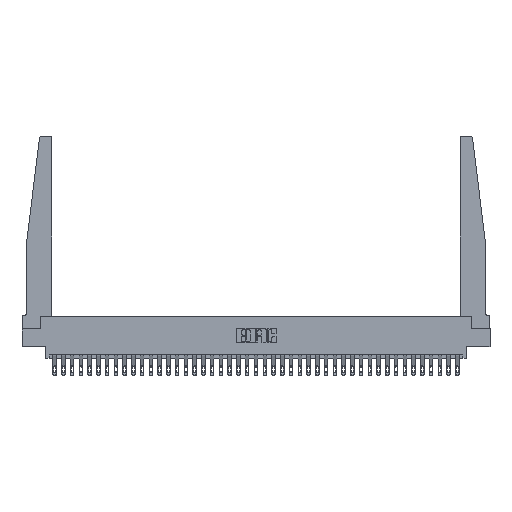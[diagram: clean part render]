
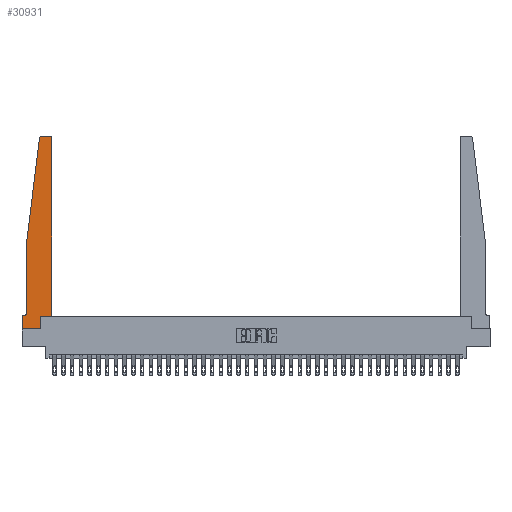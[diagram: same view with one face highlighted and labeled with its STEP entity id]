
A CAD part, top view. The second image highlights one B-rep face of the part: STEP entity #30931.
In plain terms, the highlighted planar face has unit normal (0, 0, 1).
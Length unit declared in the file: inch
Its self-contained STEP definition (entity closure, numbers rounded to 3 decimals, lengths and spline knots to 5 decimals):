
#15 = ORIENTED_EDGE ( 'NONE', *, *, #18158, .T. ) ;
#240 = CARTESIAN_POINT ( 'NONE',  ( 0.015, 0.1875, 0.37 ) ) ;
#289 = DIRECTION ( 'NONE',  ( 1., 0., 0. ) ) ;
#317 = CARTESIAN_POINT ( 'NONE',  ( 0.27653, 2.75, 0.37 ) ) ;
#432 = LINE ( 'NONE', #13810, #22222 ) ;
#491 = DIRECTION ( 'NONE',  ( 0., 0., 1. ) ) ;
#608 = EDGE_LOOP ( 'NONE', ( #12430, #9881, #7657, #9172, #32978, #2568, #4716, #7110, #5263, #15, #32462, #26759 ) ) ;
#674 = EDGE_CURVE ( 'NONE', #17049, #8147, #21334, .T. ) ;
#1508 = EDGE_CURVE ( 'NONE', #14653, #20918, #10720, .T. ) ;
#2113 = DIRECTION ( 'NONE',  ( -0.122, -0.992, 0. ) ) ;
#2166 = VECTOR ( 'NONE', #9971, 39.37008 ) ;
#2568 = ORIENTED_EDGE ( 'NONE', *, *, #34248, .T. ) ;
#2602 = EDGE_CURVE ( 'NONE', #24533, #17049, #34539, .T. ) ;
#2658 = DIRECTION ( 'NONE',  ( 0., 0., 1. ) ) ;
#4085 = VERTEX_POINT ( 'NONE', #24795 ) ;
#4716 = ORIENTED_EDGE ( 'NONE', *, *, #15577, .T. ) ;
#4764 = EDGE_CURVE ( 'NONE', #12206, #24533, #18364, .T. ) ;
#4895 = VECTOR ( 'NONE', #10423, 39.37008 ) ;
#5263 = ORIENTED_EDGE ( 'NONE', *, *, #34010, .T. ) ;
#5639 = CIRCLE ( 'NONE', #25827, 0.03 ) ;
#7110 = ORIENTED_EDGE ( 'NONE', *, *, #1508, .T. ) ;
#7355 = DIRECTION ( 'NONE',  ( 1., 0., 0. ) ) ;
#7657 = ORIENTED_EDGE ( 'NONE', *, *, #29486, .T. ) ;
#8147 = VERTEX_POINT ( 'NONE', #317 ) ;
#8255 = FACE_OUTER_BOUND ( 'NONE', #608, .T. ) ;
#8625 = CARTESIAN_POINT ( 'NONE',  ( 0., 0., 0.37 ) ) ;
#8707 = VECTOR ( 'NONE', #2113, 39.37008 ) ;
#9172 = ORIENTED_EDGE ( 'NONE', *, *, #20859, .T. ) ;
#9446 = CARTESIAN_POINT ( 'NONE',  ( 0.395, 2.75, 0.37 ) ) ;
#9881 = ORIENTED_EDGE ( 'NONE', *, *, #22931, .T. ) ;
#9971 = DIRECTION ( 'NONE',  ( -1., 0., 0. ) ) ;
#10423 = DIRECTION ( 'NONE',  ( 0., 1., 0. ) ) ;
#10720 = LINE ( 'NONE', #26637, #19489 ) ;
#12206 = VERTEX_POINT ( 'NONE', #17383 ) ;
#12224 = DIRECTION ( 'NONE',  ( 0., 0., 1. ) ) ;
#12430 = ORIENTED_EDGE ( 'NONE', *, *, #674, .T. ) ;
#13709 = VECTOR ( 'NONE', #29990, 39.37008 ) ;
#13810 = CARTESIAN_POINT ( 'NONE',  ( 0.425, 0.18, 0.37 ) ) ;
#13817 = VERTEX_POINT ( 'NONE', #22106 ) ;
#13925 = VECTOR ( 'NONE', #26921, 39.37008 ) ;
#14653 = VERTEX_POINT ( 'NONE', #8625 ) ;
#15577 = EDGE_CURVE ( 'NONE', #21917, #14653, #30214, .T. ) ;
#15705 = LINE ( 'NONE', #29074, #13925 ) ;
#16513 = LINE ( 'NONE', #25017, #29810 ) ;
#16714 = CARTESIAN_POINT ( 'NONE',  ( 0.24675, 2.72367, 0.37 ) ) ;
#16725 = CARTESIAN_POINT ( 'NONE',  ( 0., 0.1875, 0.37 ) ) ;
#17049 = VERTEX_POINT ( 'NONE', #9446 ) ;
#17383 = CARTESIAN_POINT ( 'NONE',  ( 0.425, 0.18, 0.37 ) ) ;
#18064 = VECTOR ( 'NONE', #19045, 39.37008 ) ;
#18158 = EDGE_CURVE ( 'NONE', #13817, #12206, #432, .T. ) ;
#18364 = LINE ( 'NONE', #18710, #4895 ) ;
#18710 = CARTESIAN_POINT ( 'NONE',  ( 0.425, 0.18, 0.37 ) ) ;
#19045 = DIRECTION ( 'NONE',  ( 0., -1., 0. ) ) ;
#19157 = LINE ( 'NONE', #29800, #13709 ) ;
#19233 = CARTESIAN_POINT ( 'NONE',  ( 0., 0.1875, 0.37 ) ) ;
#19489 = VECTOR ( 'NONE', #32569, 39.37008 ) ;
#20442 = CARTESIAN_POINT ( 'NONE',  ( 0.425, 2.72, 0.37 ) ) ;
#20624 = CARTESIAN_POINT ( 'NONE',  ( 0.25, 2.75, 0.37 ) ) ;
#20859 = EDGE_CURVE ( 'NONE', #4085, #24044, #15705, .T. ) ;
#20918 = VERTEX_POINT ( 'NONE', #29788 ) ;
#21334 = LINE ( 'NONE', #20624, #2166 ) ;
#21598 = AXIS2_PLACEMENT_3D ( 'NONE', #16725, #2658, #289 ) ;
#21917 = VERTEX_POINT ( 'NONE', #19233 ) ;
#22106 = CARTESIAN_POINT ( 'NONE',  ( 0.2605, 0.18, 0.37 ) ) ;
#22222 = VECTOR ( 'NONE', #33478, 39.37008 ) ;
#22291 = DIRECTION ( 'NONE',  ( 0., 1., 0. ) ) ;
#22623 = DIRECTION ( 'NONE',  ( 0., 0., -1. ) ) ;
#22931 = EDGE_CURVE ( 'NONE', #8147, #23909, #5639, .T. ) ;
#23063 = DIRECTION ( 'NONE',  ( 1., 0., 0. ) ) ;
#23225 = CARTESIAN_POINT ( 'NONE',  ( 0.27653, 2.72, 0.37 ) ) ;
#23909 = VERTEX_POINT ( 'NONE', #16714 ) ;
#24044 = VERTEX_POINT ( 'NONE', #33332 ) ;
#24533 = VERTEX_POINT ( 'NONE', #20442 ) ;
#24589 = EDGE_CURVE ( 'NONE', #24044, #27725, #29303, .T. ) ;
#24795 = CARTESIAN_POINT ( 'NONE',  ( 0.065, 1.25, 0.37 ) ) ;
#24834 = CARTESIAN_POINT ( 'NONE',  ( 0., 0., 0.37 ) ) ;
#25017 = CARTESIAN_POINT ( 'NONE',  ( 0.2605, 0.18, 0.37 ) ) ;
#25827 = AXIS2_PLACEMENT_3D ( 'NONE', #23225, #491, #23063 ) ;
#25888 = AXIS2_PLACEMENT_3D ( 'NONE', #32085, #12224, #7355 ) ;
#26637 = CARTESIAN_POINT ( 'NONE',  ( 0., 0., 0.37 ) ) ;
#26759 = ORIENTED_EDGE ( 'NONE', *, *, #2602, .T. ) ;
#26921 = DIRECTION ( 'NONE',  ( 0., -1., 0. ) ) ;
#27725 = VERTEX_POINT ( 'NONE', #240 ) ;
#28752 = CARTESIAN_POINT ( 'NONE',  ( 0.015, 0.2375, 0.37 ) ) ;
#29074 = CARTESIAN_POINT ( 'NONE',  ( 0.065, 1.25, 0.37 ) ) ;
#29197 = CARTESIAN_POINT ( 'NONE',  ( 0.065, 1.25, 0.37 ) ) ;
#29303 = CIRCLE ( 'NONE', #29895, 0.05 ) ;
#29486 = EDGE_CURVE ( 'NONE', #23909, #4085, #29553, .T. ) ;
#29553 = LINE ( 'NONE', #29197, #8707 ) ;
#29788 = CARTESIAN_POINT ( 'NONE',  ( 0.2605, 0., 0.37 ) ) ;
#29800 = CARTESIAN_POINT ( 'NONE',  ( 0.065, 0.1875, 0.37 ) ) ;
#29810 = VECTOR ( 'NONE', #22291, 39.37008 ) ;
#29895 = AXIS2_PLACEMENT_3D ( 'NONE', #28752, #22623, #33627 ) ;
#29990 = DIRECTION ( 'NONE',  ( -1., 0., 0. ) ) ;
#30214 = LINE ( 'NONE', #24834, #18064 ) ;
#30262 = PLANE ( 'NONE',  #21598 ) ;
#30931 = ADVANCED_FACE ( 'NONE', ( #8255 ), #30262, .T. ) ;
#32085 = CARTESIAN_POINT ( 'NONE',  ( 0.395, 2.72, 0.37 ) ) ;
#32462 = ORIENTED_EDGE ( 'NONE', *, *, #4764, .T. ) ;
#32569 = DIRECTION ( 'NONE',  ( 1., 0., 0. ) ) ;
#32978 = ORIENTED_EDGE ( 'NONE', *, *, #24589, .T. ) ;
#33332 = CARTESIAN_POINT ( 'NONE',  ( 0.065, 0.2375, 0.37 ) ) ;
#33478 = DIRECTION ( 'NONE',  ( 1., 0., 0. ) ) ;
#33627 = DIRECTION ( 'NONE',  ( -1., 0., 0. ) ) ;
#34010 = EDGE_CURVE ( 'NONE', #20918, #13817, #16513, .T. ) ;
#34248 = EDGE_CURVE ( 'NONE', #27725, #21917, #19157, .T. ) ;
#34539 = CIRCLE ( 'NONE', #25888, 0.03 ) ;
